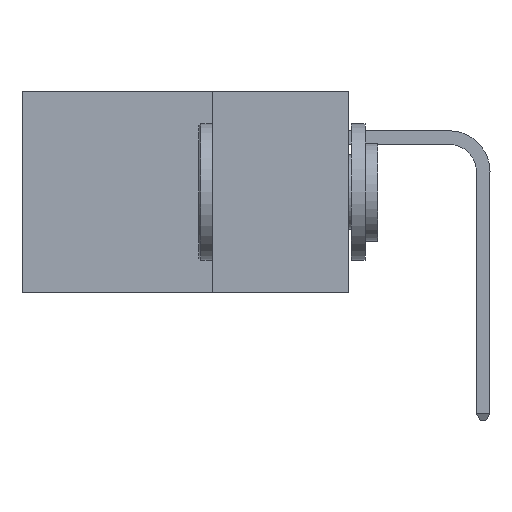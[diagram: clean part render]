
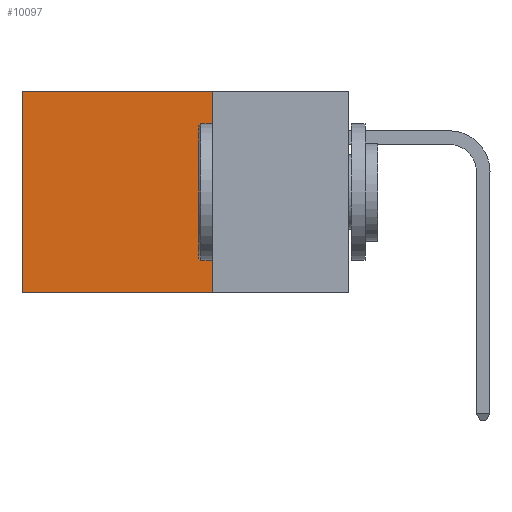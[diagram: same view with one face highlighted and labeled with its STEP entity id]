
A CAD part, left-side view. The second image highlights one B-rep face of the part: STEP entity #10097.
In plain terms, the highlighted planar face has unit normal (-1, 0, 0).
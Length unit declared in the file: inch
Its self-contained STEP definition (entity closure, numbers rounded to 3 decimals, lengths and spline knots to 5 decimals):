
#217 = EDGE_CURVE ( 'NONE', #7062, #12395, #4766, .T. ) ;
#1726 = VECTOR ( 'NONE', #11212, 39.37008 ) ;
#1881 = CARTESIAN_POINT ( 'NONE',  ( 0.2875, 0.25, 0. ) ) ;
#2050 = VECTOR ( 'NONE', #9157, 39.37008 ) ;
#3240 = CARTESIAN_POINT ( 'NONE',  ( 0.2875, 0.25, -0.37 ) ) ;
#3648 = VECTOR ( 'NONE', #17323, 39.37008 ) ;
#4576 = EDGE_CURVE ( 'NONE', #18081, #5556, #10142, .T. ) ;
#4766 = LINE ( 'NONE', #9949, #14429 ) ;
#5556 = VERTEX_POINT ( 'NONE', #19841 ) ;
#6612 = PLANE ( 'NONE',  #15618 ) ;
#6673 = ORIENTED_EDGE ( 'NONE', *, *, #17673, .T. ) ;
#7062 = VERTEX_POINT ( 'NONE', #13076 ) ;
#7562 = FACE_OUTER_BOUND ( 'NONE', #16449, .T. ) ;
#7877 = CARTESIAN_POINT ( 'NONE',  ( 0.2875, 0.6, 0. ) ) ;
#7903 = CARTESIAN_POINT ( 'NONE',  ( 0.2875, 0.6, 0. ) ) ;
#9157 = DIRECTION ( 'NONE',  ( 0., 1., 0. ) ) ;
#9778 = EDGE_CURVE ( 'NONE', #12395, #5556, #13588, .T. ) ;
#9949 = CARTESIAN_POINT ( 'NONE',  ( 0.2875, 0.25, 0. ) ) ;
#10097 = ADVANCED_FACE ( 'NONE', ( #7562 ), #6612, .F. ) ;
#10142 = LINE ( 'NONE', #7877, #3648 ) ;
#11041 = ORIENTED_EDGE ( 'NONE', *, *, #217, .F. ) ;
#11212 = DIRECTION ( 'NONE',  ( 0., 1., 0. ) ) ;
#12395 = VERTEX_POINT ( 'NONE', #3240 ) ;
#12511 = CARTESIAN_POINT ( 'NONE',  ( 0.2875, 0.25, -0.37 ) ) ;
#12735 = ORIENTED_EDGE ( 'NONE', *, *, #4576, .T. ) ;
#12832 = DIRECTION ( 'NONE',  ( 0., 0., -1. ) ) ;
#13076 = CARTESIAN_POINT ( 'NONE',  ( 0.2875, 0.25, 0. ) ) ;
#13588 = LINE ( 'NONE', #12511, #2050 ) ;
#14031 = LINE ( 'NONE', #18756, #1726 ) ;
#14429 = VECTOR ( 'NONE', #17462, 39.37008 ) ;
#15501 = ORIENTED_EDGE ( 'NONE', *, *, #9778, .F. ) ;
#15618 = AXIS2_PLACEMENT_3D ( 'NONE', #1881, #17396, #12832 ) ;
#16449 = EDGE_LOOP ( 'NONE', ( #12735, #15501, #11041, #6673 ) ) ;
#17323 = DIRECTION ( 'NONE',  ( 0., 0., -1. ) ) ;
#17396 = DIRECTION ( 'NONE',  ( 1., 0., 0. ) ) ;
#17462 = DIRECTION ( 'NONE',  ( 0., 0., -1. ) ) ;
#17673 = EDGE_CURVE ( 'NONE', #7062, #18081, #14031, .T. ) ;
#18081 = VERTEX_POINT ( 'NONE', #7903 ) ;
#18756 = CARTESIAN_POINT ( 'NONE',  ( 0.2875, 0.25, 0. ) ) ;
#19841 = CARTESIAN_POINT ( 'NONE',  ( 0.2875, 0.6, -0.37 ) ) ;
